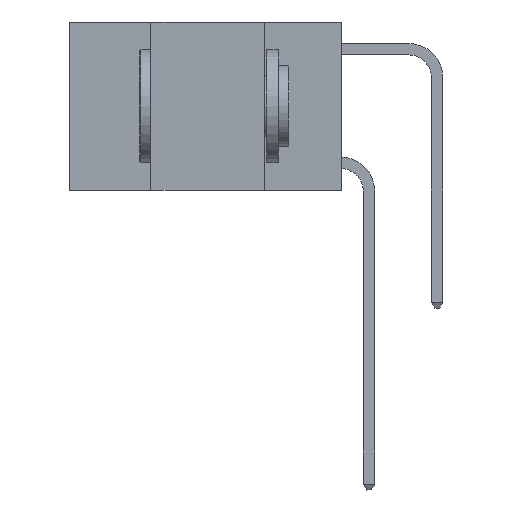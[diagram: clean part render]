
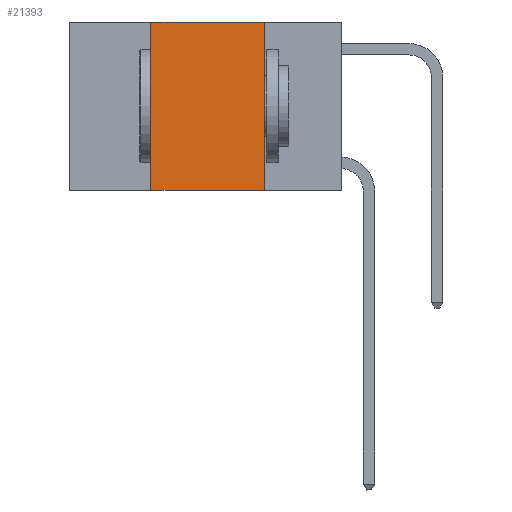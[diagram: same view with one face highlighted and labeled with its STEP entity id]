
A CAD part, left-side view. The second image highlights one B-rep face of the part: STEP entity #21393.
In plain terms, the highlighted planar face has unit normal (-1, 0, 0).
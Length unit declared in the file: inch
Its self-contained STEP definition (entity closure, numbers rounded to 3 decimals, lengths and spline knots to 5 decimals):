
#865 = CARTESIAN_POINT ( 'NONE',  ( 0., 0.42, 0. ) ) ;
#1760 = DIRECTION ( 'NONE',  ( 1., 0., 0. ) ) ;
#1816 = DIRECTION ( 'NONE',  ( 0., 0., 1. ) ) ;
#1913 = CARTESIAN_POINT ( 'NONE',  ( 0., 0.6, 0. ) ) ;
#1941 = ORIENTED_EDGE ( 'NONE', *, *, #18554, .F. ) ;
#3283 = PLANE ( 'NONE',  #17578 ) ;
#3356 = VECTOR ( 'NONE', #1816, 39.37008 ) ;
#3810 = LINE ( 'NONE', #5462, #3356 ) ;
#4406 = VECTOR ( 'NONE', #20319, 39.37008 ) ;
#4605 = CARTESIAN_POINT ( 'NONE',  ( 0., 0.6, 0. ) ) ;
#4619 = ORIENTED_EDGE ( 'NONE', *, *, #9979, .F. ) ;
#5164 = DIRECTION ( 'NONE',  ( 0., 0., -1. ) ) ;
#5462 = CARTESIAN_POINT ( 'NONE',  ( 0., 0.42, 0. ) ) ;
#6469 = LINE ( 'NONE', #22412, #20883 ) ;
#6823 = CARTESIAN_POINT ( 'NONE',  ( 0., 0.17, -0.37 ) ) ;
#7546 = LINE ( 'NONE', #1913, #4406 ) ;
#7742 = CARTESIAN_POINT ( 'NONE',  ( 0., 0.42, -0.37 ) ) ;
#7752 = DIRECTION ( 'NONE',  ( 0., -1., 0. ) ) ;
#8554 = CARTESIAN_POINT ( 'NONE',  ( 0., 0.17, 0. ) ) ;
#9979 = EDGE_CURVE ( 'NONE', #11261, #19980, #15632, .T. ) ;
#11261 = VERTEX_POINT ( 'NONE', #16709 ) ;
#11762 = VERTEX_POINT ( 'NONE', #7742 ) ;
#13091 = ORIENTED_EDGE ( 'NONE', *, *, #22369, .F. ) ;
#14144 = VERTEX_POINT ( 'NONE', #865 ) ;
#15632 = LINE ( 'NONE', #8554, #19000 ) ;
#15748 = DIRECTION ( 'NONE',  ( 0., 0., -1. ) ) ;
#15938 = EDGE_LOOP ( 'NONE', ( #4619, #1941, #13091, #20272 ) ) ;
#16709 = CARTESIAN_POINT ( 'NONE',  ( 0., 0.17, 0. ) ) ;
#17578 = AXIS2_PLACEMENT_3D ( 'NONE', #4605, #1760, #5164 ) ;
#18554 = EDGE_CURVE ( 'NONE', #14144, #11261, #7546, .T. ) ;
#19000 = VECTOR ( 'NONE', #15748, 39.37008 ) ;
#19832 = EDGE_CURVE ( 'NONE', #11762, #19980, #6469, .T. ) ;
#19980 = VERTEX_POINT ( 'NONE', #6823 ) ;
#20272 = ORIENTED_EDGE ( 'NONE', *, *, #19832, .T. ) ;
#20319 = DIRECTION ( 'NONE',  ( 0., -1., 0. ) ) ;
#20883 = VECTOR ( 'NONE', #7752, 39.37008 ) ;
#21229 = FACE_OUTER_BOUND ( 'NONE', #15938, .T. ) ;
#21393 = ADVANCED_FACE ( 'NONE', ( #21229 ), #3283, .F. ) ;
#22369 = EDGE_CURVE ( 'NONE', #11762, #14144, #3810, .T. ) ;
#22412 = CARTESIAN_POINT ( 'NONE',  ( 0., 0.6, -0.37 ) ) ;
